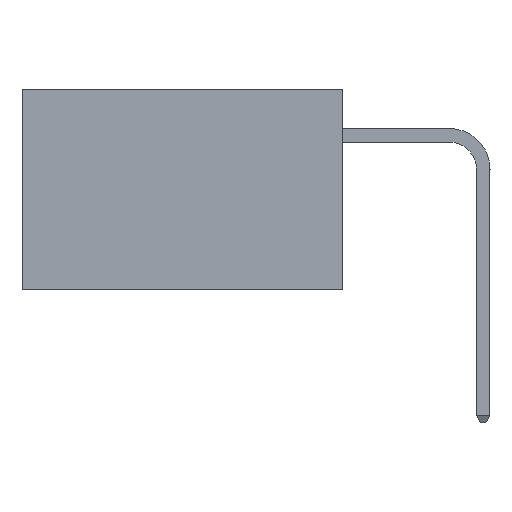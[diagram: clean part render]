
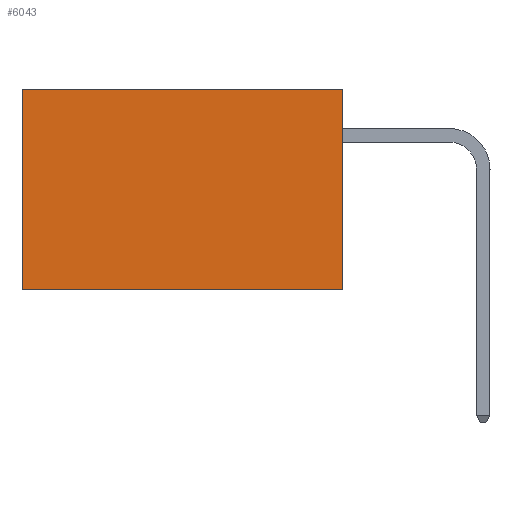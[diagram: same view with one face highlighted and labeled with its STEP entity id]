
A CAD part, left-side view. The second image highlights one B-rep face of the part: STEP entity #6043.
In plain terms, the highlighted planar face has unit normal (-1, 0, 0).
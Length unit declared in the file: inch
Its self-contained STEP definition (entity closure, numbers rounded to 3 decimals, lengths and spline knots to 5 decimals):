
#2117 = DIRECTION ( 'NONE',  ( 0., 0., -1. ) ) ;
#2897 = LINE ( 'NONE', #11856, #8948 ) ;
#3032 = VERTEX_POINT ( 'NONE', #4766 ) ;
#4028 = FACE_OUTER_BOUND ( 'NONE', #15245, .T. ) ;
#4121 = DIRECTION ( 'NONE',  ( 0., 1., 0. ) ) ;
#4348 = AXIS2_PLACEMENT_3D ( 'NONE', #4991, #5181, #5155 ) ;
#4485 = PLANE ( 'NONE',  #4348 ) ;
#4719 = VERTEX_POINT ( 'NONE', #14463 ) ;
#4766 = CARTESIAN_POINT ( 'NONE',  ( 0.277, 0., 0. ) ) ;
#4991 = CARTESIAN_POINT ( 'NONE',  ( 0.277, 0., -0.37 ) ) ;
#5155 = DIRECTION ( 'NONE',  ( 0., 0., -1. ) ) ;
#5181 = DIRECTION ( 'NONE',  ( 1., 0., 0. ) ) ;
#5508 = EDGE_CURVE ( 'NONE', #10558, #6130, #9096, .T. ) ;
#5967 = CARTESIAN_POINT ( 'NONE',  ( 0.277, 0.59, -0.37 ) ) ;
#6043 = ADVANCED_FACE ( 'NONE', ( #4028 ), #4485, .F. ) ;
#6130 = VERTEX_POINT ( 'NONE', #5967 ) ;
#6566 = EDGE_CURVE ( 'NONE', #3032, #10558, #15267, .T. ) ;
#8396 = ORIENTED_EDGE ( 'NONE', *, *, #14949, .F. ) ;
#8556 = ORIENTED_EDGE ( 'NONE', *, *, #5508, .T. ) ;
#8858 = CARTESIAN_POINT ( 'NONE',  ( 0.277, 0., -0.37 ) ) ;
#8863 = VECTOR ( 'NONE', #14856, 39.37008 ) ;
#8948 = VECTOR ( 'NONE', #2117, 39.37008 ) ;
#9096 = LINE ( 'NONE', #9114, #12366 ) ;
#9114 = CARTESIAN_POINT ( 'NONE',  ( 0.277, 0.59, -0.37 ) ) ;
#9914 = ORIENTED_EDGE ( 'NONE', *, *, #12371, .F. ) ;
#10525 = ORIENTED_EDGE ( 'NONE', *, *, #6566, .T. ) ;
#10558 = VERTEX_POINT ( 'NONE', #15026 ) ;
#11158 = LINE ( 'NONE', #8858, #13584 ) ;
#11856 = CARTESIAN_POINT ( 'NONE',  ( 0.277, 0., -0.37 ) ) ;
#11874 = DIRECTION ( 'NONE',  ( 0., 0., -1. ) ) ;
#12366 = VECTOR ( 'NONE', #11874, 39.37008 ) ;
#12371 = EDGE_CURVE ( 'NONE', #3032, #4719, #2897, .T. ) ;
#13584 = VECTOR ( 'NONE', #4121, 39.37008 ) ;
#14463 = CARTESIAN_POINT ( 'NONE',  ( 0.277, 0., -0.37 ) ) ;
#14856 = DIRECTION ( 'NONE',  ( 0., 1., 0. ) ) ;
#14949 = EDGE_CURVE ( 'NONE', #4719, #6130, #11158, .T. ) ;
#15026 = CARTESIAN_POINT ( 'NONE',  ( 0.277, 0.59, 0. ) ) ;
#15037 = CARTESIAN_POINT ( 'NONE',  ( 0.277, 0., 0. ) ) ;
#15245 = EDGE_LOOP ( 'NONE', ( #8556, #8396, #9914, #10525 ) ) ;
#15267 = LINE ( 'NONE', #15037, #8863 ) ;
